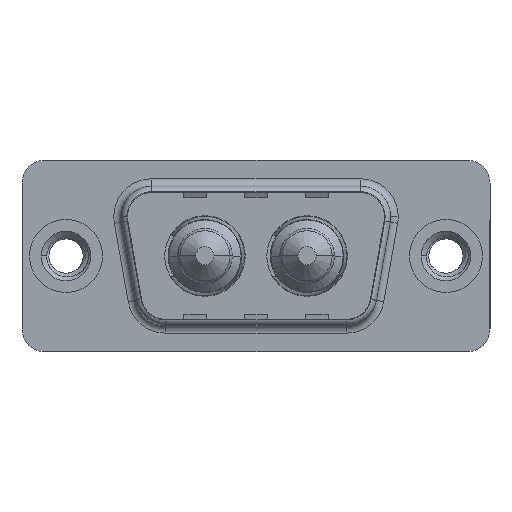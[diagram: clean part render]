
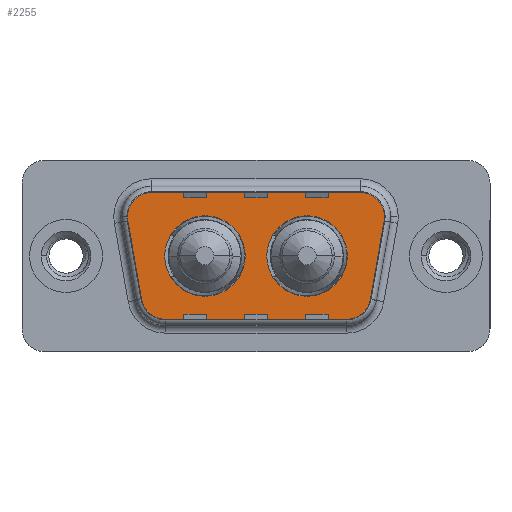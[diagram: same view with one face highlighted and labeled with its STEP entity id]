
A CAD part, top view. The second image highlights one B-rep face of the part: STEP entity #2255.
In plain terms, the highlighted planar face has unit normal (0, 0, 1).
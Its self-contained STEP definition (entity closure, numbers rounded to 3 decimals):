
#90 = CIRCLE ( 'NONE', #9142, 2.65 ) ;
#278 = CIRCLE ( 'NONE', #6969, 2. ) ;
#291 = AXIS2_PLACEMENT_3D ( 'NONE', #2969, #9279, #3880 ) ;
#440 = AXIS2_PLACEMENT_3D ( 'NONE', #10260, #4826, #11193 ) ;
#449 = VECTOR ( 'NONE', #10645, 1000. ) ;
#479 = DIRECTION ( 'NONE',  ( 0., 0., 1. ) ) ;
#768 = DIRECTION ( 'NONE',  ( 1., 0., 0. ) ) ;
#771 = AXIS2_PLACEMENT_3D ( 'NONE', #9160, #900, #10103 ) ;
#900 = DIRECTION ( 'NONE',  ( 0., 0., 1. ) ) ;
#907 = CARTESIAN_POINT ( 'NONE',  ( 6.49, 0., 0. ) ) ;
#927 = VERTEX_POINT ( 'NONE', #11311 ) ;
#969 = FACE_BOUND ( 'NONE', #4959, .T. ) ;
#1151 = EDGE_CURVE ( 'NONE', #11680, #1311, #1891, .T. ) ;
#1311 = VERTEX_POINT ( 'NONE', #9983 ) ;
#1442 = CARTESIAN_POINT ( 'NONE',  ( 15.86, 0., 0. ) ) ;
#1443 = VERTEX_POINT ( 'NONE', #10522 ) ;
#1883 = CARTESIAN_POINT ( 'NONE',  ( 11.79, 0., 0. ) ) ;
#1891 = LINE ( 'NONE', #10141, #449 ) ;
#2129 = ORIENTED_EDGE ( 'NONE', *, *, #8924, .F. ) ;
#2217 = CARTESIAN_POINT ( 'NONE',  ( 19.564, 2.9, 0. ) ) ;
#2255 = ADVANCED_FACE ( 'NONE', ( #5711, #969, #10867 ), #2467, .T. ) ;
#2325 = VECTOR ( 'NONE', #7154, 1000. ) ;
#2467 = PLANE ( 'NONE',  #771 ) ;
#2847 = EDGE_CURVE ( 'NONE', #7825, #1443, #3609, .T. ) ;
#2937 = ORIENTED_EDGE ( 'NONE', *, *, #7455, .F. ) ;
#2957 = ORIENTED_EDGE ( 'NONE', *, *, #7412, .T. ) ;
#2969 = CARTESIAN_POINT ( 'NONE',  ( 9.14, 0., 0. ) ) ;
#3029 = DIRECTION ( 'NONE',  ( 0., 0., 1. ) ) ;
#3264 = CARTESIAN_POINT ( 'NONE',  ( 3.466, 2.553, 0. ) ) ;
#3310 = EDGE_CURVE ( 'NONE', #10225, #4797, #90, .T. ) ;
#3342 = ORIENTED_EDGE ( 'NONE', *, *, #5344, .T. ) ;
#3514 = CARTESIAN_POINT ( 'NONE',  ( 5.436, 2.9, 0. ) ) ;
#3609 = LINE ( 'NONE', #10434, #10258 ) ;
#3726 = AXIS2_PLACEMENT_3D ( 'NONE', #7893, #8296, #10473 ) ;
#3880 = DIRECTION ( 'NONE',  ( 1., 0., 0. ) ) ;
#3959 = CIRCLE ( 'NONE', #7531, 2.65 ) ;
#4108 = EDGE_LOOP ( 'NONE', ( #2937, #9955 ) ) ;
#4395 = AXIS2_PLACEMENT_3D ( 'NONE', #2217, #11218, #4550 ) ;
#4423 = DIRECTION ( 'NONE',  ( 1., 0., 0. ) ) ;
#4532 = CARTESIAN_POINT ( 'NONE',  ( 15.86, 0., 0. ) ) ;
#4550 = DIRECTION ( 'NONE',  ( -1., 0., 0. ) ) ;
#4557 = LINE ( 'NONE', #9565, #6919 ) ;
#4648 = EDGE_CURVE ( 'NONE', #9373, #8731, #4994, .T. ) ;
#4716 = ORIENTED_EDGE ( 'NONE', *, *, #10017, .T. ) ;
#4733 = CARTESIAN_POINT ( 'NONE',  ( 6.459, -2.9, 0. ) ) ;
#4797 = VERTEX_POINT ( 'NONE', #6431 ) ;
#4826 = DIRECTION ( 'NONE',  ( 0., 0., 1. ) ) ;
#4935 = ORIENTED_EDGE ( 'NONE', *, *, #2847, .T. ) ;
#4959 = EDGE_LOOP ( 'NONE', ( #11244, #2129 ) ) ;
#4994 = CIRCLE ( 'NONE', #4395, 2. ) ;
#5071 = DIRECTION ( 'NONE',  ( 1., 0., 0. ) ) ;
#5124 = CARTESIAN_POINT ( 'NONE',  ( 6.459, -4.9, 0. ) ) ;
#5130 = ORIENTED_EDGE ( 'NONE', *, *, #6370, .T. ) ;
#5274 = CARTESIAN_POINT ( 'NONE',  ( 20.511, -3.247, 0. ) ) ;
#5334 = CIRCLE ( 'NONE', #440, 2.65 ) ;
#5344 = EDGE_CURVE ( 'NONE', #1311, #9373, #5671, .T. ) ;
#5630 = CARTESIAN_POINT ( 'NONE',  ( 21.564, 2.9, 0. ) ) ;
#5671 = CIRCLE ( 'NONE', #3726, 2. ) ;
#5711 = FACE_BOUND ( 'NONE', #4108, .T. ) ;
#5752 = AXIS2_PLACEMENT_3D ( 'NONE', #4733, #8252, #8301 ) ;
#5835 = EDGE_CURVE ( 'NONE', #8731, #10579, #4557, .T. ) ;
#5921 = VERTEX_POINT ( 'NONE', #1883 ) ;
#5962 = DIRECTION ( 'NONE',  ( 0., 0., 1. ) ) ;
#6126 = CARTESIAN_POINT ( 'NONE',  ( 18.541, -2.9, 0. ) ) ;
#6370 = EDGE_CURVE ( 'NONE', #927, #11680, #9916, .T. ) ;
#6431 = CARTESIAN_POINT ( 'NONE',  ( 18.51, 0., 0. ) ) ;
#6441 = DIRECTION ( 'NONE',  ( -1., 0., 0. ) ) ;
#6607 = CIRCLE ( 'NONE', #5752, 2. ) ;
#6641 = EDGE_CURVE ( 'NONE', #9846, #927, #11632, .T. ) ;
#6919 = VECTOR ( 'NONE', #6441, 1000. ) ;
#6969 = AXIS2_PLACEMENT_3D ( 'NONE', #3514, #9838, #4423 ) ;
#7154 = DIRECTION ( 'NONE',  ( 1., 0., 0. ) ) ;
#7412 = EDGE_CURVE ( 'NONE', #1443, #9846, #6607, .T. ) ;
#7455 = EDGE_CURVE ( 'NONE', #4797, #10225, #3959, .T. ) ;
#7531 = AXIS2_PLACEMENT_3D ( 'NONE', #4532, #479, #768 ) ;
#7825 = VERTEX_POINT ( 'NONE', #3264 ) ;
#7893 = CARTESIAN_POINT ( 'NONE',  ( 19.564, 2.9, 0. ) ) ;
#8029 = ORIENTED_EDGE ( 'NONE', *, *, #6641, .T. ) ;
#8252 = DIRECTION ( 'NONE',  ( 0., 0., 1. ) ) ;
#8253 = ORIENTED_EDGE ( 'NONE', *, *, #4648, .T. ) ;
#8296 = DIRECTION ( 'NONE',  ( 0., 0., 1. ) ) ;
#8301 = DIRECTION ( 'NONE',  ( -1., 0., 0. ) ) ;
#8469 = AXIS2_PLACEMENT_3D ( 'NONE', #6126, #3029, #9446 ) ;
#8731 = VERTEX_POINT ( 'NONE', #8899 ) ;
#8772 = CARTESIAN_POINT ( 'NONE',  ( 13.21, 0., 0. ) ) ;
#8899 = CARTESIAN_POINT ( 'NONE',  ( 19.564, 4.9, 0. ) ) ;
#8924 = EDGE_CURVE ( 'NONE', #10101, #5921, #5334, .T. ) ;
#9113 = ORIENTED_EDGE ( 'NONE', *, *, #1151, .T. ) ;
#9142 = AXIS2_PLACEMENT_3D ( 'NONE', #1442, #5962, #5071 ) ;
#9160 = CARTESIAN_POINT ( 'NONE',  ( 18.541, -2.9, 0. ) ) ;
#9279 = DIRECTION ( 'NONE',  ( 0., 0., 1. ) ) ;
#9300 = CARTESIAN_POINT ( 'NONE',  ( 6.459, -4.9, 0. ) ) ;
#9373 = VERTEX_POINT ( 'NONE', #5630 ) ;
#9446 = DIRECTION ( 'NONE',  ( 1., 0., 0. ) ) ;
#9565 = CARTESIAN_POINT ( 'NONE',  ( 5.436, 4.9, 0. ) ) ;
#9724 = DIRECTION ( 'NONE',  ( 0.174, -0.985, 0. ) ) ;
#9838 = DIRECTION ( 'NONE',  ( 0., 0., 1. ) ) ;
#9846 = VERTEX_POINT ( 'NONE', #5124 ) ;
#9916 = CIRCLE ( 'NONE', #8469, 2. ) ;
#9955 = ORIENTED_EDGE ( 'NONE', *, *, #3310, .F. ) ;
#9983 = CARTESIAN_POINT ( 'NONE',  ( 21.534, 2.553, 0. ) ) ;
#10017 = EDGE_CURVE ( 'NONE', #10579, #7825, #278, .T. ) ;
#10076 = EDGE_LOOP ( 'NONE', ( #5130, #9113, #3342, #8253, #11066, #4716, #4935, #2957, #8029 ) ) ;
#10101 = VERTEX_POINT ( 'NONE', #907 ) ;
#10103 = DIRECTION ( 'NONE',  ( 1., 0., 0. ) ) ;
#10141 = CARTESIAN_POINT ( 'NONE',  ( 21.534, 2.553, 0. ) ) ;
#10157 = CIRCLE ( 'NONE', #291, 2.65 ) ;
#10178 = CARTESIAN_POINT ( 'NONE',  ( 5.436, 4.9, 0. ) ) ;
#10225 = VERTEX_POINT ( 'NONE', #8772 ) ;
#10258 = VECTOR ( 'NONE', #9724, 1000. ) ;
#10260 = CARTESIAN_POINT ( 'NONE',  ( 9.14, 0., 0. ) ) ;
#10434 = CARTESIAN_POINT ( 'NONE',  ( 3.466, 2.553, 0. ) ) ;
#10473 = DIRECTION ( 'NONE',  ( -1., 0., 0. ) ) ;
#10522 = CARTESIAN_POINT ( 'NONE',  ( 4.489, -3.247, 0. ) ) ;
#10573 = EDGE_CURVE ( 'NONE', #5921, #10101, #10157, .T. ) ;
#10579 = VERTEX_POINT ( 'NONE', #10178 ) ;
#10645 = DIRECTION ( 'NONE',  ( 0.174, 0.985, 0. ) ) ;
#10867 = FACE_OUTER_BOUND ( 'NONE', #10076, .T. ) ;
#11066 = ORIENTED_EDGE ( 'NONE', *, *, #5835, .T. ) ;
#11193 = DIRECTION ( 'NONE',  ( 1., 0., 0. ) ) ;
#11218 = DIRECTION ( 'NONE',  ( 0., 0., 1. ) ) ;
#11244 = ORIENTED_EDGE ( 'NONE', *, *, #10573, .F. ) ;
#11311 = CARTESIAN_POINT ( 'NONE',  ( 18.541, -4.9, 0. ) ) ;
#11632 = LINE ( 'NONE', #9300, #2325 ) ;
#11680 = VERTEX_POINT ( 'NONE', #5274 ) ;
